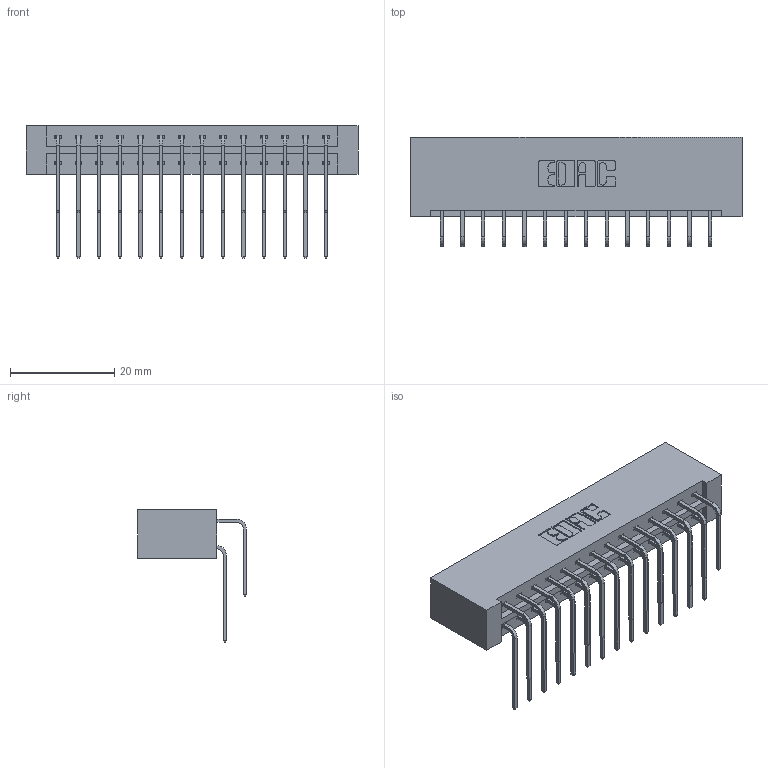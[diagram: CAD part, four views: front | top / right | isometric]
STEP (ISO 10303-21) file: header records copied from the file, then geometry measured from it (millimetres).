
FILE_DESCRIPTION (( 'STEP AP203' ), '1' );
FILE_NAME ('333-028-559-201.STEP', '2018-08-02T15:52:50', ( '' ), ( '' ), 'SwSTEP 2.0', 'SolidWorks 2016', '' );
FILE_SCHEMA (( 'CONFIG_CONTROL_DESIGN' ));
Length unit declared in the file: inch
Products named in the file (4): 333 Part_Lugless; 345-292-001_558 559 Tail - 1; 345-292-001_559 Tail - 2; 333-028-559-201
Assembly tree (29 placements, depth 2):
  333-028-559-201
    333 Part_Lugless
    345-292-001_558 559 Tail - 1  x14
    345-292-001_559 Tail - 2  x14
Bounding box: 63.73 x 20.9 x 25.53 mm (x, y, z)
Volume: 7038.2 mm3; surface area: 8849 mm2
Topology: 29 solids, 29 shells, 1618 faces, 4795 edges, 3158 vertices
Faces by surface type: plane 1130, cylinder 488
Entity records: 14135 total; most frequent: CARTESIAN_POINT 2425, ORIENTED_EDGE 2310, DIRECTION 2095, EDGE_CURVE 1155, VECTOR 995, LINE 995, VERTEX_POINT 766, AXIS2_PLACEMENT_3D 550
